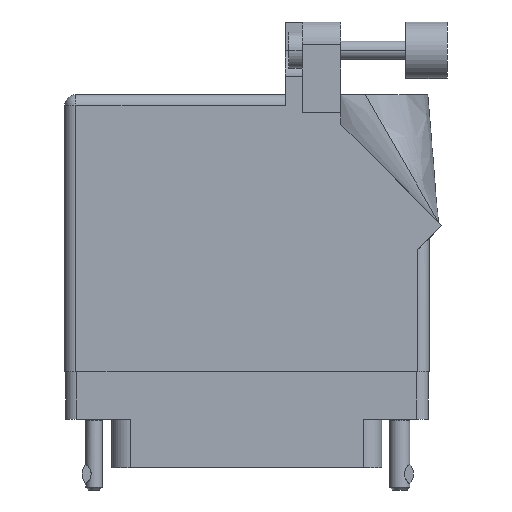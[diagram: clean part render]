
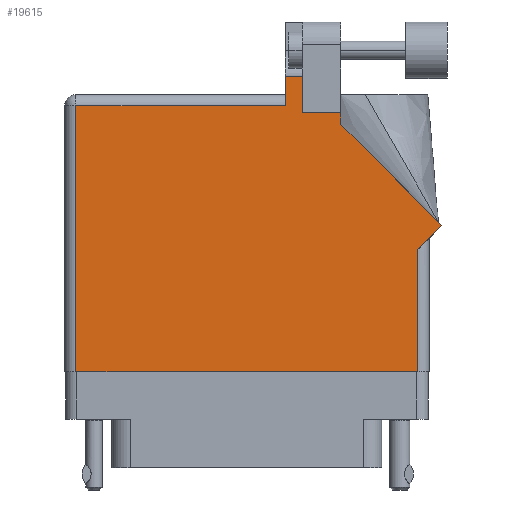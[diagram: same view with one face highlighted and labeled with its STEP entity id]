
A CAD part, front view. The second image highlights one B-rep face of the part: STEP entity #19615.
In plain terms, the highlighted face is planar.
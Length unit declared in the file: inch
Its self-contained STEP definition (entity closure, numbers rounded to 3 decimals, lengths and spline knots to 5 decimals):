
#477 = VERTEX_POINT ( 'NONE', #23962 ) ;
#1003 = DIRECTION ( 'NONE',  ( 0., 1., 0. ) ) ;
#1939 = CARTESIAN_POINT ( 'NONE',  ( 1.948, 0.675, 0. ) ) ;
#1963 = EDGE_CURVE ( 'NONE', #26291, #9586, #20912, .T. ) ;
#3453 = EDGE_CURVE ( 'NONE', #31465, #17842, #34287, .T. ) ;
#3582 = DIRECTION ( 'NONE',  ( 0., -1., 0. ) ) ;
#4139 = LINE ( 'NONE', #22356, #17075 ) ;
#4148 = CARTESIAN_POINT ( 'NONE',  ( 2.01, 0.737, 0. ) ) ;
#4456 = ORIENTED_EDGE ( 'NONE', *, *, #25398, .T. ) ;
#5009 = VERTEX_POINT ( 'NONE', #5931 ) ;
#5239 = ORIENTED_EDGE ( 'NONE', *, *, #28775, .T. ) ;
#5807 = VERTEX_POINT ( 'NONE', #45639 ) ;
#5931 = CARTESIAN_POINT ( 'NONE',  ( 1.311, 1.43, 0. ) ) ;
#6672 = VECTOR ( 'NONE', #21614, 39.37008 ) ;
#7035 = CARTESIAN_POINT ( 'NONE',  ( 0.062, 0., 0. ) ) ;
#8395 = CARTESIAN_POINT ( 'NONE',  ( 1.217, 1.468, 0. ) ) ;
#9216 = VECTOR ( 'NONE', #32607, 39.37008 ) ;
#9586 = VERTEX_POINT ( 'NONE', #37214 ) ;
#10129 = CARTESIAN_POINT ( 'NONE',  ( 0., 0., 0. ) ) ;
#10352 = ORIENTED_EDGE ( 'NONE', *, *, #16481, .T. ) ;
#10577 = FACE_OUTER_BOUND ( 'NONE', #28661, .T. ) ;
#10721 = VERTEX_POINT ( 'NONE', #18168 ) ;
#11209 = VERTEX_POINT ( 'NONE', #8395 ) ;
#11726 = DIRECTION ( 'NONE',  ( 0.707, 0.707, 0. ) ) ;
#12352 = CARTESIAN_POINT ( 'NONE',  ( 1.311, 1.43, 0. ) ) ;
#12673 = EDGE_CURVE ( 'NONE', #10721, #5807, #14666, .T. ) ;
#14666 = LINE ( 'NONE', #38952, #42746 ) ;
#15134 = CARTESIAN_POINT ( 'NONE',  ( 1.217, 1.53, 0. ) ) ;
#15140 = CARTESIAN_POINT ( 'NONE',  ( 1.948, 0.737, 0. ) ) ;
#15370 = LINE ( 'NONE', #7035, #33598 ) ;
#15467 = VECTOR ( 'NONE', #26098, 39.37008 ) ;
#16341 = DIRECTION ( 'NONE',  ( -1., 0., 0. ) ) ;
#16376 = CARTESIAN_POINT ( 'NONE',  ( 1.524, 1.36442, 0. ) ) ;
#16384 = CARTESIAN_POINT ( 'NONE',  ( 0.062, 0., 0. ) ) ;
#16481 = EDGE_CURVE ( 'NONE', #47618, #5009, #18387, .T. ) ;
#17075 = VECTOR ( 'NONE', #22836, 39.37008 ) ;
#17266 = LINE ( 'NONE', #12352, #32514 ) ;
#17287 = VECTOR ( 'NONE', #38988, 39.37008 ) ;
#17842 = VERTEX_POINT ( 'NONE', #32071 ) ;
#18125 = EDGE_CURVE ( 'NONE', #9586, #477, #4139, .T. ) ;
#18168 = CARTESIAN_POINT ( 'NONE',  ( 1.311, 1.6315, 0. ) ) ;
#18387 = LINE ( 'NONE', #22789, #15467 ) ;
#19615 = ADVANCED_FACE ( 'NONE', ( #10577 ), #39892, .F. ) ;
#19980 = EDGE_CURVE ( 'NONE', #5807, #11209, #35770, .T. ) ;
#20912 = LINE ( 'NONE', #4148, #38489 ) ;
#21561 = CARTESIAN_POINT ( 'NONE',  ( 0., 1.53, 0. ) ) ;
#21614 = DIRECTION ( 'NONE',  ( 1., 0., 0. ) ) ;
#22356 = CARTESIAN_POINT ( 'NONE',  ( 2.08071, 0.80771, 0. ) ) ;
#22789 = CARTESIAN_POINT ( 'NONE',  ( 1.524, 1.43, 0. ) ) ;
#22836 = DIRECTION ( 'NONE',  ( -0.707, 0.707, 0. ) ) ;
#23332 = ORIENTED_EDGE ( 'NONE', *, *, #3453, .T. ) ;
#23613 = ORIENTED_EDGE ( 'NONE', *, *, #47074, .T. ) ;
#23962 = CARTESIAN_POINT ( 'NONE',  ( 1.524, 1.36442, 0. ) ) ;
#24676 = DIRECTION ( 'NONE',  ( 0., 0., -1. ) ) ;
#25398 = EDGE_CURVE ( 'NONE', #5009, #10721, #17266, .T. ) ;
#26098 = DIRECTION ( 'NONE',  ( -1., 0., 0. ) ) ;
#26291 = VERTEX_POINT ( 'NONE', #1939 ) ;
#26569 = CARTESIAN_POINT ( 'NONE',  ( 0.062, 1.468, 0. ) ) ;
#27214 = VECTOR ( 'NONE', #43701, 39.37008 ) ;
#28661 = EDGE_LOOP ( 'NONE', ( #4456, #43762, #28697, #37871, #5239, #23332, #23613, #32513, #47702, #46566, #10352 ) ) ;
#28697 = ORIENTED_EDGE ( 'NONE', *, *, #19980, .T. ) ;
#28775 = EDGE_CURVE ( 'NONE', #28777, #31465, #15370, .T. ) ;
#28777 = VERTEX_POINT ( 'NONE', #26569 ) ;
#31465 = VERTEX_POINT ( 'NONE', #16384 ) ;
#31606 = VECTOR ( 'NONE', #34324, 39.37008 ) ;
#32071 = CARTESIAN_POINT ( 'NONE',  ( 1.948, 0., 0. ) ) ;
#32513 = ORIENTED_EDGE ( 'NONE', *, *, #1963, .T. ) ;
#32514 = VECTOR ( 'NONE', #1003, 39.37008 ) ;
#32607 = DIRECTION ( 'NONE',  ( -1., 0., 0. ) ) ;
#33182 = CARTESIAN_POINT ( 'NONE',  ( 1.524, 1.43, 0. ) ) ;
#33598 = VECTOR ( 'NONE', #3582, 39.37008 ) ;
#34287 = LINE ( 'NONE', #10129, #6672 ) ;
#34324 = DIRECTION ( 'NONE',  ( 0., -1., 0. ) ) ;
#35770 = LINE ( 'NONE', #15134, #31606 ) ;
#37214 = CARTESIAN_POINT ( 'NONE',  ( 2.08071, 0.80771, 0. ) ) ;
#37871 = ORIENTED_EDGE ( 'NONE', *, *, #45126, .T. ) ;
#38382 = LINE ( 'NONE', #16376, #17287 ) ;
#38489 = VECTOR ( 'NONE', #11726, 39.37008 ) ;
#38952 = CARTESIAN_POINT ( 'NONE',  ( 1.64177, 1.6315, 0. ) ) ;
#38988 = DIRECTION ( 'NONE',  ( 0., 1., 0. ) ) ;
#39563 = DIRECTION ( 'NONE',  ( -1., 0., 0. ) ) ;
#39892 = PLANE ( 'NONE',  #44222 ) ;
#40116 = LINE ( 'NONE', #15140, #27214 ) ;
#41308 = EDGE_CURVE ( 'NONE', #477, #47618, #38382, .T. ) ;
#42746 = VECTOR ( 'NONE', #16341, 39.37008 ) ;
#43191 = LINE ( 'NONE', #48058, #9216 ) ;
#43701 = DIRECTION ( 'NONE',  ( 0., 1., 0. ) ) ;
#43762 = ORIENTED_EDGE ( 'NONE', *, *, #12673, .T. ) ;
#44222 = AXIS2_PLACEMENT_3D ( 'NONE', #21561, #24676, #39563 ) ;
#45126 = EDGE_CURVE ( 'NONE', #11209, #28777, #43191, .T. ) ;
#45639 = CARTESIAN_POINT ( 'NONE',  ( 1.217, 1.6315, 0. ) ) ;
#46566 = ORIENTED_EDGE ( 'NONE', *, *, #41308, .T. ) ;
#47074 = EDGE_CURVE ( 'NONE', #17842, #26291, #40116, .T. ) ;
#47618 = VERTEX_POINT ( 'NONE', #33182 ) ;
#47702 = ORIENTED_EDGE ( 'NONE', *, *, #18125, .T. ) ;
#48058 = CARTESIAN_POINT ( 'NONE',  ( 0., 1.468, 0. ) ) ;
